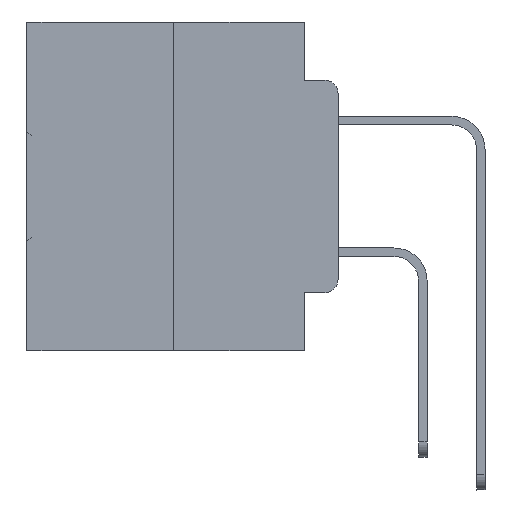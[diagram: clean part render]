
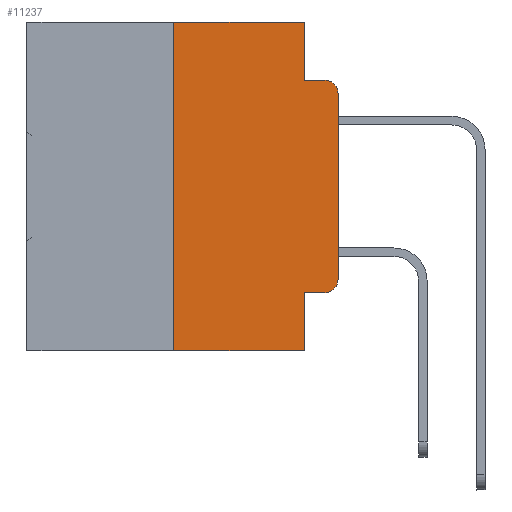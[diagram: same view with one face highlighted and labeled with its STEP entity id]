
A CAD part, left-side view. The second image highlights one B-rep face of the part: STEP entity #11237.
In plain terms, the highlighted planar face has unit normal (-1, 0, 0).
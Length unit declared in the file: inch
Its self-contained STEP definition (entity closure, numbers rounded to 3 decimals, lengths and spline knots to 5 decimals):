
#117 = VERTEX_POINT ( 'NONE', #28567 ) ;
#329 = CARTESIAN_POINT ( 'NONE',  ( 0., 0.473, 0. ) ) ;
#2007 = CARTESIAN_POINT ( 'NONE',  ( 0., 0., -0.3915 ) ) ;
#2036 = ORIENTED_EDGE ( 'NONE', *, *, #19223, .F. ) ;
#2346 = CARTESIAN_POINT ( 'NONE',  ( 0., 0., -0.1085 ) ) ;
#3137 = EDGE_CURVE ( 'NONE', #28365, #23416, #22130, .T. ) ;
#3186 = DIRECTION ( 'NONE',  ( 0., 0., -1. ) ) ;
#3972 = ORIENTED_EDGE ( 'NONE', *, *, #16929, .T. ) ;
#5761 = EDGE_CURVE ( 'NONE', #117, #21440, #32926, .T. ) ;
#6302 = DIRECTION ( 'NONE',  ( 0., 0., -1. ) ) ;
#6433 = VECTOR ( 'NONE', #34104, 39.37008 ) ;
#6907 = AXIS2_PLACEMENT_3D ( 'NONE', #29774, #13417, #32441 ) ;
#7405 = VERTEX_POINT ( 'NONE', #23379 ) ;
#7868 = CARTESIAN_POINT ( 'NONE',  ( 0., 0.051, -0.5 ) ) ;
#7892 = CARTESIAN_POINT ( 'NONE',  ( 0., 0., 0. ) ) ;
#8047 = EDGE_CURVE ( 'NONE', #23416, #26417, #19695, .T. ) ;
#8095 = DIRECTION ( 'NONE',  ( 0., -1., 0. ) ) ;
#8187 = DIRECTION ( 'NONE',  ( 0., -1., 0. ) ) ;
#8825 = VERTEX_POINT ( 'NONE', #24541 ) ;
#9203 = CARTESIAN_POINT ( 'NONE',  ( 0., 0.02, -0.3915 ) ) ;
#10160 = EDGE_CURVE ( 'NONE', #26417, #23827, #27240, .T. ) ;
#10318 = AXIS2_PLACEMENT_3D ( 'NONE', #329, #19876, #3186 ) ;
#10368 = CARTESIAN_POINT ( 'NONE',  ( 0., 0.051, 0. ) ) ;
#10505 = CARTESIAN_POINT ( 'NONE',  ( 0., 0.25, 0. ) ) ;
#10680 = FACE_OUTER_BOUND ( 'NONE', #31076, .T. ) ;
#11237 = ADVANCED_FACE ( 'NONE', ( #10680 ), #33384, .F. ) ;
#11690 = ORIENTED_EDGE ( 'NONE', *, *, #17909, .F. ) ;
#12038 = DIRECTION ( 'NONE',  ( 0., 0., -1. ) ) ;
#12385 = AXIS2_PLACEMENT_3D ( 'NONE', #9203, #28471, #12038 ) ;
#12655 = CARTESIAN_POINT ( 'NONE',  ( 0., 0.051, -0.0885 ) ) ;
#13038 = ORIENTED_EDGE ( 'NONE', *, *, #28447, .F. ) ;
#13417 = DIRECTION ( 'NONE',  ( -1., 0., 0. ) ) ;
#13436 = VECTOR ( 'NONE', #15434, 39.37008 ) ;
#13670 = CARTESIAN_POINT ( 'NONE',  ( 0., 0.473, 0. ) ) ;
#13683 = ORIENTED_EDGE ( 'NONE', *, *, #23853, .F. ) ;
#14405 = LINE ( 'NONE', #22940, #35233 ) ;
#14883 = VECTOR ( 'NONE', #8187, 39.37008 ) ;
#15434 = DIRECTION ( 'NONE',  ( 0., -1., 0. ) ) ;
#16339 = DIRECTION ( 'NONE',  ( 0., 0., 1. ) ) ;
#16929 = EDGE_CURVE ( 'NONE', #23827, #7405, #17710, .T. ) ;
#17710 = CIRCLE ( 'NONE', #6907, 0.02 ) ;
#17909 = EDGE_CURVE ( 'NONE', #23759, #8825, #14405, .T. ) ;
#17987 = VECTOR ( 'NONE', #24690, 39.37008 ) ;
#18192 = ORIENTED_EDGE ( 'NONE', *, *, #8047, .T. ) ;
#18554 = EDGE_CURVE ( 'NONE', #28365, #21440, #27616, .T. ) ;
#18976 = DIRECTION ( 'NONE',  ( 0., 0., 1. ) ) ;
#19223 = EDGE_CURVE ( 'NONE', #8825, #7405, #35137, .T. ) ;
#19695 = CIRCLE ( 'NONE', #12385, 0.02 ) ;
#19876 = DIRECTION ( 'NONE',  ( 1., 0., 0. ) ) ;
#19935 = CARTESIAN_POINT ( 'NONE',  ( 0., 0.02, -0.4115 ) ) ;
#21285 = ORIENTED_EDGE ( 'NONE', *, *, #10160, .T. ) ;
#21440 = VERTEX_POINT ( 'NONE', #7868 ) ;
#21769 = CARTESIAN_POINT ( 'NONE',  ( 0., 0.473, -0.5 ) ) ;
#22130 = LINE ( 'NONE', #27485, #14883 ) ;
#22940 = CARTESIAN_POINT ( 'NONE',  ( 0., 0.051, 0. ) ) ;
#23379 = CARTESIAN_POINT ( 'NONE',  ( 0., 0.02, -0.0885 ) ) ;
#23416 = VERTEX_POINT ( 'NONE', #19935 ) ;
#23759 = VERTEX_POINT ( 'NONE', #10368 ) ;
#23827 = VERTEX_POINT ( 'NONE', #2346 ) ;
#23853 = EDGE_CURVE ( 'NONE', #27837, #23759, #32376, .T. ) ;
#23975 = ORIENTED_EDGE ( 'NONE', *, *, #3137, .T. ) ;
#24541 = CARTESIAN_POINT ( 'NONE',  ( 0., 0.051, -0.0885 ) ) ;
#24690 = DIRECTION ( 'NONE',  ( 0., -1., 0. ) ) ;
#25270 = ORIENTED_EDGE ( 'NONE', *, *, #5761, .T. ) ;
#25826 = VECTOR ( 'NONE', #8095, 39.37008 ) ;
#26402 = VECTOR ( 'NONE', #16339, 39.37008 ) ;
#26417 = VERTEX_POINT ( 'NONE', #2007 ) ;
#26748 = CARTESIAN_POINT ( 'NONE',  ( 0., 0.051, -0.4115 ) ) ;
#27017 = LINE ( 'NONE', #10505, #33313 ) ;
#27240 = LINE ( 'NONE', #7892, #26402 ) ;
#27485 = CARTESIAN_POINT ( 'NONE',  ( 0., 0.051, -0.4115 ) ) ;
#27616 = LINE ( 'NONE', #31411, #6433 ) ;
#27837 = VERTEX_POINT ( 'NONE', #32517 ) ;
#28365 = VERTEX_POINT ( 'NONE', #26748 ) ;
#28447 = EDGE_CURVE ( 'NONE', #117, #27837, #27017, .T. ) ;
#28471 = DIRECTION ( 'NONE',  ( -1., 0., 0. ) ) ;
#28567 = CARTESIAN_POINT ( 'NONE',  ( 0., 0.25, -0.5 ) ) ;
#29774 = CARTESIAN_POINT ( 'NONE',  ( 0., 0.02, -0.1085 ) ) ;
#31076 = EDGE_LOOP ( 'NONE', ( #21285, #3972, #2036, #11690, #13683, #13038, #25270, #31744, #23975, #18192 ) ) ;
#31411 = CARTESIAN_POINT ( 'NONE',  ( 0., 0.051, 0. ) ) ;
#31744 = ORIENTED_EDGE ( 'NONE', *, *, #18554, .F. ) ;
#32376 = LINE ( 'NONE', #13670, #17987 ) ;
#32441 = DIRECTION ( 'NONE',  ( 0., 0., -1. ) ) ;
#32517 = CARTESIAN_POINT ( 'NONE',  ( 0., 0.25, 0. ) ) ;
#32926 = LINE ( 'NONE', #21769, #25826 ) ;
#33313 = VECTOR ( 'NONE', #18976, 39.37008 ) ;
#33384 = PLANE ( 'NONE',  #10318 ) ;
#34104 = DIRECTION ( 'NONE',  ( 0., 0., -1. ) ) ;
#35137 = LINE ( 'NONE', #12655, #13436 ) ;
#35233 = VECTOR ( 'NONE', #6302, 39.37008 ) ;
